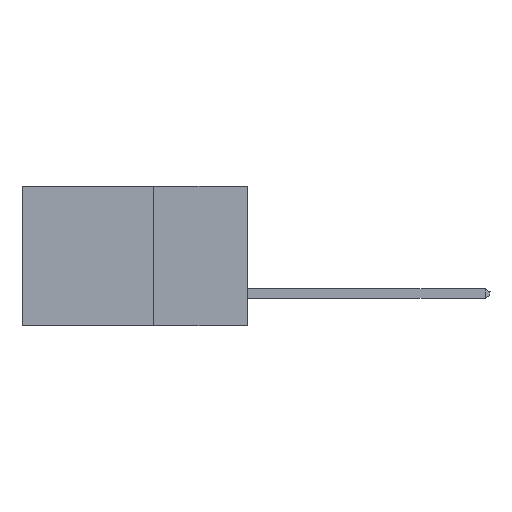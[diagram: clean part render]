
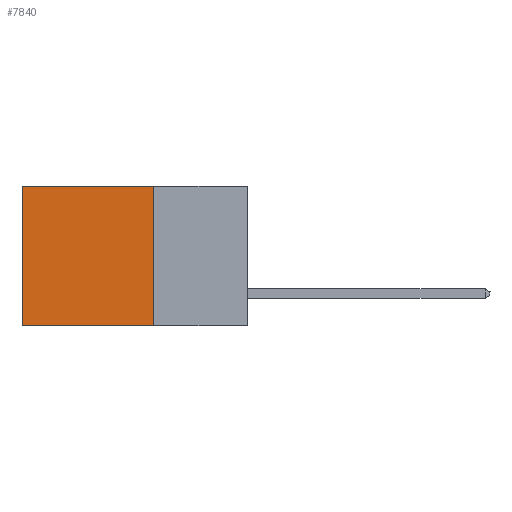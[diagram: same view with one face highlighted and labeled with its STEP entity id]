
A CAD part, left-side view. The second image highlights one B-rep face of the part: STEP entity #7840.
In plain terms, the highlighted planar face has unit normal (-1, 0, 0).
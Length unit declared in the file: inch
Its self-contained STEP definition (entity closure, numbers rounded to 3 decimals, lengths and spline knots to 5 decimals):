
#559 = EDGE_CURVE ( 'NONE', #1422, #9114, #6161, .T. ) ;
#795 = EDGE_LOOP ( 'NONE', ( #11353, #4355, #8355, #3075 ) ) ;
#1035 = PLANE ( 'NONE',  #11122 ) ;
#1422 = VERTEX_POINT ( 'NONE', #7963 ) ;
#2129 = EDGE_CURVE ( 'NONE', #9114, #5387, #4491, .T. ) ;
#2919 = LINE ( 'NONE', #4870, #10970 ) ;
#3075 = ORIENTED_EDGE ( 'NONE', *, *, #6771, .T. ) ;
#3331 = VECTOR ( 'NONE', #7183, 39.37008 ) ;
#3918 = LINE ( 'NONE', #4841, #7476 ) ;
#4355 = ORIENTED_EDGE ( 'NONE', *, *, #2129, .F. ) ;
#4491 = LINE ( 'NONE', #7498, #4817 ) ;
#4817 = VECTOR ( 'NONE', #11409, 39.37008 ) ;
#4841 = CARTESIAN_POINT ( 'NONE',  ( 0.2615, 0.25, 0. ) ) ;
#4870 = CARTESIAN_POINT ( 'NONE',  ( 0.2615, 0.6, -0.37 ) ) ;
#5208 = CARTESIAN_POINT ( 'NONE',  ( 0.2615, 0.25, -0.37 ) ) ;
#5387 = VERTEX_POINT ( 'NONE', #7743 ) ;
#5884 = CARTESIAN_POINT ( 'NONE',  ( 0.2615, 0.25, -0.37 ) ) ;
#6161 = LINE ( 'NONE', #5208, #3331 ) ;
#6707 = CARTESIAN_POINT ( 'NONE',  ( 0.2615, 0.25, -0.37 ) ) ;
#6771 = EDGE_CURVE ( 'NONE', #1422, #8162, #3918, .T. ) ;
#7183 = DIRECTION ( 'NONE',  ( 0., 0., -1. ) ) ;
#7313 = EDGE_CURVE ( 'NONE', #8162, #5387, #2919, .T. ) ;
#7476 = VECTOR ( 'NONE', #11740, 39.37008 ) ;
#7498 = CARTESIAN_POINT ( 'NONE',  ( 0.2615, 0.25, -0.37 ) ) ;
#7725 = DIRECTION ( 'NONE',  ( 0., 0., -1. ) ) ;
#7743 = CARTESIAN_POINT ( 'NONE',  ( 0.2615, 0.6, -0.37 ) ) ;
#7840 = ADVANCED_FACE ( 'NONE', ( #10869 ), #1035, .F. ) ;
#7963 = CARTESIAN_POINT ( 'NONE',  ( 0.2615, 0.25, 0. ) ) ;
#8162 = VERTEX_POINT ( 'NONE', #10470 ) ;
#8355 = ORIENTED_EDGE ( 'NONE', *, *, #559, .F. ) ;
#9114 = VERTEX_POINT ( 'NONE', #5884 ) ;
#9904 = DIRECTION ( 'NONE',  ( 0., 0., -1. ) ) ;
#10470 = CARTESIAN_POINT ( 'NONE',  ( 0.2615, 0.6, 0. ) ) ;
#10614 = DIRECTION ( 'NONE',  ( 1., 0., 0. ) ) ;
#10869 = FACE_OUTER_BOUND ( 'NONE', #795, .T. ) ;
#10970 = VECTOR ( 'NONE', #9904, 39.37008 ) ;
#11122 = AXIS2_PLACEMENT_3D ( 'NONE', #6707, #10614, #7725 ) ;
#11353 = ORIENTED_EDGE ( 'NONE', *, *, #7313, .T. ) ;
#11409 = DIRECTION ( 'NONE',  ( 0., 1., 0. ) ) ;
#11740 = DIRECTION ( 'NONE',  ( 0., 1., 0. ) ) ;
